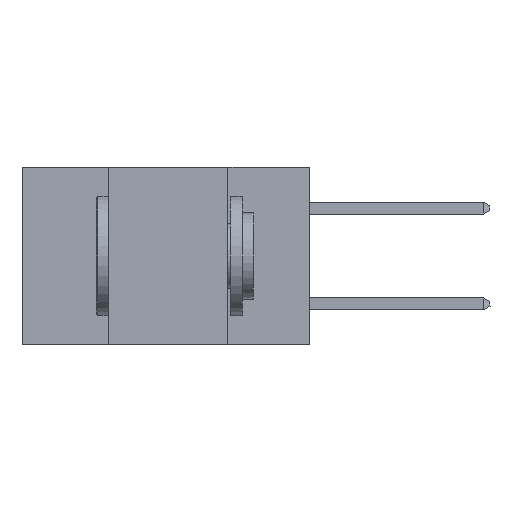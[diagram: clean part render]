
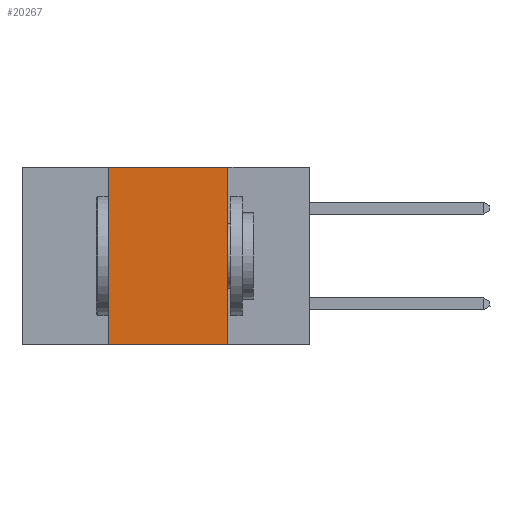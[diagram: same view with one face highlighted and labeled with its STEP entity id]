
A CAD part, left-side view. The second image highlights one B-rep face of the part: STEP entity #20267.
In plain terms, the highlighted planar face has unit normal (-1, 0, 0).
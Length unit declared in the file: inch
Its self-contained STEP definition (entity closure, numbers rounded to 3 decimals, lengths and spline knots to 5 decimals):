
#1774 = VERTEX_POINT ( 'NONE', #22066 ) ;
#3654 = CARTESIAN_POINT ( 'NONE',  ( 0., 0.6, 0. ) ) ;
#3757 = VERTEX_POINT ( 'NONE', #7550 ) ;
#3760 = VECTOR ( 'NONE', #6453, 39.37008 ) ;
#4518 = CARTESIAN_POINT ( 'NONE',  ( 0., 0.17, 0. ) ) ;
#5563 = DIRECTION ( 'NONE',  ( 1., 0., 0. ) ) ;
#6453 = DIRECTION ( 'NONE',  ( 0., 0., -1. ) ) ;
#6957 = VERTEX_POINT ( 'NONE', #15062 ) ;
#7280 = EDGE_CURVE ( 'NONE', #3757, #6957, #9146, .T. ) ;
#7288 = ORIENTED_EDGE ( 'NONE', *, *, #7280, .F. ) ;
#7550 = CARTESIAN_POINT ( 'NONE',  ( 0., 0.42, 0. ) ) ;
#7770 = DIRECTION ( 'NONE',  ( 0., 0., 1. ) ) ;
#7915 = DIRECTION ( 'NONE',  ( 0., -1., 0. ) ) ;
#8591 = VECTOR ( 'NONE', #14207, 39.37008 ) ;
#9146 = LINE ( 'NONE', #21047, #8591 ) ;
#9508 = EDGE_CURVE ( 'NONE', #20802, #1774, #14432, .T. ) ;
#11715 = ORIENTED_EDGE ( 'NONE', *, *, #9508, .T. ) ;
#12252 = EDGE_CURVE ( 'NONE', #6957, #1774, #23215, .T. ) ;
#12465 = LINE ( 'NONE', #18391, #17185 ) ;
#13262 = ORIENTED_EDGE ( 'NONE', *, *, #12252, .F. ) ;
#14207 = DIRECTION ( 'NONE',  ( 0., -1., 0. ) ) ;
#14432 = LINE ( 'NONE', #15044, #18504 ) ;
#14603 = PLANE ( 'NONE',  #19526 ) ;
#15044 = CARTESIAN_POINT ( 'NONE',  ( 0., 0.6, -0.37 ) ) ;
#15062 = CARTESIAN_POINT ( 'NONE',  ( 0., 0.17, 0. ) ) ;
#16587 = EDGE_CURVE ( 'NONE', #20802, #3757, #12465, .T. ) ;
#17185 = VECTOR ( 'NONE', #7770, 39.37008 ) ;
#18104 = DIRECTION ( 'NONE',  ( 0., 0., -1. ) ) ;
#18121 = ORIENTED_EDGE ( 'NONE', *, *, #16587, .F. ) ;
#18391 = CARTESIAN_POINT ( 'NONE',  ( 0., 0.42, 0. ) ) ;
#18504 = VECTOR ( 'NONE', #7915, 39.37008 ) ;
#19475 = FACE_OUTER_BOUND ( 'NONE', #20427, .T. ) ;
#19526 = AXIS2_PLACEMENT_3D ( 'NONE', #3654, #5563, #18104 ) ;
#20267 = ADVANCED_FACE ( 'NONE', ( #19475 ), #14603, .F. ) ;
#20427 = EDGE_LOOP ( 'NONE', ( #13262, #7288, #18121, #11715 ) ) ;
#20802 = VERTEX_POINT ( 'NONE', #21105 ) ;
#21047 = CARTESIAN_POINT ( 'NONE',  ( 0., 0.6, 0. ) ) ;
#21105 = CARTESIAN_POINT ( 'NONE',  ( 0., 0.42, -0.37 ) ) ;
#22066 = CARTESIAN_POINT ( 'NONE',  ( 0., 0.17, -0.37 ) ) ;
#23215 = LINE ( 'NONE', #4518, #3760 ) ;
